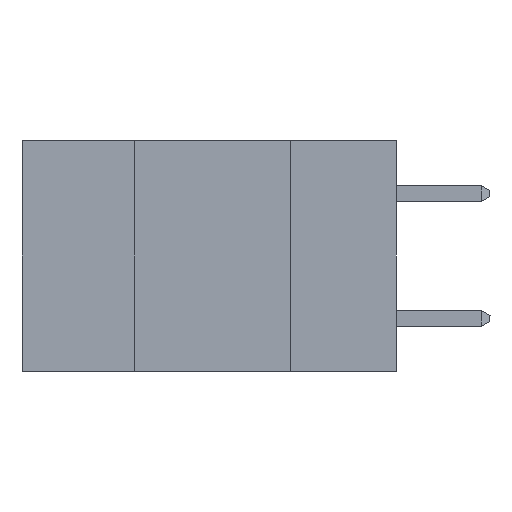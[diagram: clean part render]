
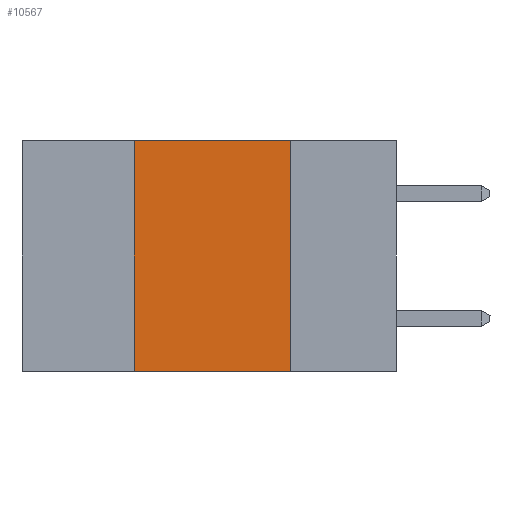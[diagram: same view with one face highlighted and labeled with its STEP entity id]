
A CAD part, left-side view. The second image highlights one B-rep face of the part: STEP entity #10567.
In plain terms, the highlighted planar face has unit normal (-1, 0, 0).
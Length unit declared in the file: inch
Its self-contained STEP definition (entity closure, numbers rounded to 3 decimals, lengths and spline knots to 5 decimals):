
#840 = ORIENTED_EDGE ( 'NONE', *, *, #3061, .F. ) ;
#1158 = VECTOR ( 'NONE', #10155, 39.37008 ) ;
#1576 = EDGE_CURVE ( 'NONE', #3337, #13101, #3315, .T. ) ;
#1811 = DIRECTION ( 'NONE',  ( 1., 0., 0. ) ) ;
#1862 = DIRECTION ( 'NONE',  ( 0., -1., 0. ) ) ;
#2804 = LINE ( 'NONE', #4386, #14371 ) ;
#3061 = EDGE_CURVE ( 'NONE', #13101, #4170, #9679, .T. ) ;
#3315 = LINE ( 'NONE', #7250, #12308 ) ;
#3337 = VERTEX_POINT ( 'NONE', #4596 ) ;
#3882 = DIRECTION ( 'NONE',  ( 0., 0., 1. ) ) ;
#4099 = ORIENTED_EDGE ( 'NONE', *, *, #13879, .F. ) ;
#4170 = VERTEX_POINT ( 'NONE', #13341 ) ;
#4386 = CARTESIAN_POINT ( 'NONE',  ( 0., 0.42, -0.37 ) ) ;
#4596 = CARTESIAN_POINT ( 'NONE',  ( 0., 0.42, 0. ) ) ;
#5164 = CARTESIAN_POINT ( 'NONE',  ( 0., 0.6, -0.37 ) ) ;
#6465 = CARTESIAN_POINT ( 'NONE',  ( 0., 0.17, 0. ) ) ;
#7061 = CARTESIAN_POINT ( 'NONE',  ( 0., 0.17, -0.37 ) ) ;
#7083 = ORIENTED_EDGE ( 'NONE', *, *, #12387, .T. ) ;
#7250 = CARTESIAN_POINT ( 'NONE',  ( 0., 0.6, 0. ) ) ;
#7267 = DIRECTION ( 'NONE',  ( 0., -1., 0. ) ) ;
#8451 = CARTESIAN_POINT ( 'NONE',  ( 0., 0.6, 0. ) ) ;
#9593 = DIRECTION ( 'NONE',  ( 0., 0., -1. ) ) ;
#9679 = LINE ( 'NONE', #7061, #1158 ) ;
#10155 = DIRECTION ( 'NONE',  ( 0., 0., -1. ) ) ;
#10295 = AXIS2_PLACEMENT_3D ( 'NONE', #8451, #1811, #9593 ) ;
#10567 = ADVANCED_FACE ( 'NONE', ( #14463 ), #10692, .F. ) ;
#10692 = PLANE ( 'NONE',  #10295 ) ;
#12308 = VECTOR ( 'NONE', #7267, 39.37008 ) ;
#12387 = EDGE_CURVE ( 'NONE', #13995, #4170, #13251, .T. ) ;
#12472 = CARTESIAN_POINT ( 'NONE',  ( 0., 0.42, -0.37 ) ) ;
#12806 = ORIENTED_EDGE ( 'NONE', *, *, #1576, .F. ) ;
#13101 = VERTEX_POINT ( 'NONE', #6465 ) ;
#13251 = LINE ( 'NONE', #5164, #13583 ) ;
#13341 = CARTESIAN_POINT ( 'NONE',  ( 0., 0.17, -0.37 ) ) ;
#13583 = VECTOR ( 'NONE', #1862, 39.37008 ) ;
#13879 = EDGE_CURVE ( 'NONE', #13995, #3337, #2804, .T. ) ;
#13995 = VERTEX_POINT ( 'NONE', #12472 ) ;
#14346 = EDGE_LOOP ( 'NONE', ( #840, #12806, #4099, #7083 ) ) ;
#14371 = VECTOR ( 'NONE', #3882, 39.37008 ) ;
#14463 = FACE_OUTER_BOUND ( 'NONE', #14346, .T. ) ;
